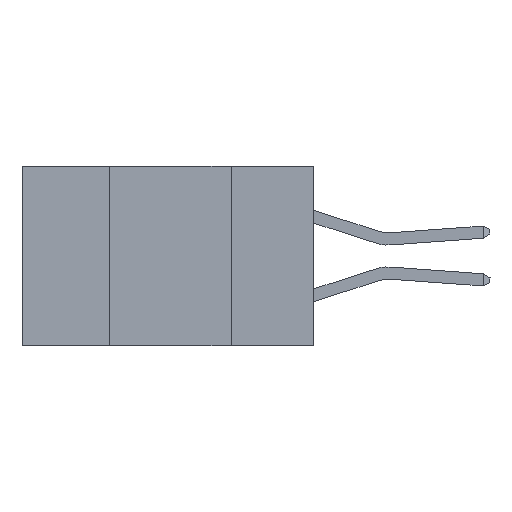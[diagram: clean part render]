
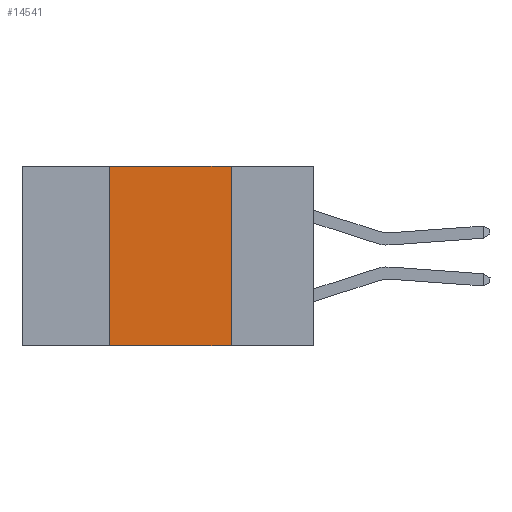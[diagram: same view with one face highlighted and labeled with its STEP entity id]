
A CAD part, left-side view. The second image highlights one B-rep face of the part: STEP entity #14541.
In plain terms, the highlighted planar face has unit normal (-1, 0, 0).
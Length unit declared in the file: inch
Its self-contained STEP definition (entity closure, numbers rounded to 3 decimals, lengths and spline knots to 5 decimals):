
#114 = CARTESIAN_POINT ( 'NONE',  ( 0., 0.42, 0. ) ) ;
#957 = CARTESIAN_POINT ( 'NONE',  ( 0., 0.6, 0. ) ) ;
#1025 = LINE ( 'NONE', #11012, #9658 ) ;
#1291 = VECTOR ( 'NONE', #13780, 39.37008 ) ;
#1461 = DIRECTION ( 'NONE',  ( 0., 0., -1. ) ) ;
#3761 = LINE ( 'NONE', #13973, #9531 ) ;
#5796 = EDGE_CURVE ( 'NONE', #7577, #7219, #10593, .T. ) ;
#5825 = DIRECTION ( 'NONE',  ( 1., 0., 0. ) ) ;
#6589 = EDGE_CURVE ( 'NONE', #7577, #11306, #13295, .T. ) ;
#7219 = VERTEX_POINT ( 'NONE', #9376 ) ;
#7380 = EDGE_CURVE ( 'NONE', #11321, #7219, #3761, .T. ) ;
#7577 = VERTEX_POINT ( 'NONE', #10891 ) ;
#7833 = CARTESIAN_POINT ( 'NONE',  ( 0., 0.42, 0. ) ) ;
#8542 = DIRECTION ( 'NONE',  ( 0., 0., 1. ) ) ;
#8641 = AXIS2_PLACEMENT_3D ( 'NONE', #957, #5825, #13574 ) ;
#8946 = CARTESIAN_POINT ( 'NONE',  ( 0., 0.17, 0. ) ) ;
#9052 = EDGE_CURVE ( 'NONE', #11306, #11321, #1025, .T. ) ;
#9376 = CARTESIAN_POINT ( 'NONE',  ( 0., 0.17, -0.37 ) ) ;
#9531 = VECTOR ( 'NONE', #1461, 39.37008 ) ;
#9658 = VECTOR ( 'NONE', #14293, 39.37008 ) ;
#10530 = CARTESIAN_POINT ( 'NONE',  ( 0., 0.6, -0.37 ) ) ;
#10593 = LINE ( 'NONE', #10530, #1291 ) ;
#10736 = VECTOR ( 'NONE', #8542, 39.37008 ) ;
#10891 = CARTESIAN_POINT ( 'NONE',  ( 0., 0.42, -0.37 ) ) ;
#10918 = FACE_OUTER_BOUND ( 'NONE', #11100, .T. ) ;
#11012 = CARTESIAN_POINT ( 'NONE',  ( 0., 0.6, 0. ) ) ;
#11100 = EDGE_LOOP ( 'NONE', ( #11796, #13339, #12402, #13402 ) ) ;
#11306 = VERTEX_POINT ( 'NONE', #7833 ) ;
#11321 = VERTEX_POINT ( 'NONE', #8946 ) ;
#11355 = PLANE ( 'NONE',  #8641 ) ;
#11796 = ORIENTED_EDGE ( 'NONE', *, *, #7380, .F. ) ;
#12402 = ORIENTED_EDGE ( 'NONE', *, *, #6589, .F. ) ;
#13295 = LINE ( 'NONE', #114, #10736 ) ;
#13339 = ORIENTED_EDGE ( 'NONE', *, *, #9052, .F. ) ;
#13402 = ORIENTED_EDGE ( 'NONE', *, *, #5796, .T. ) ;
#13574 = DIRECTION ( 'NONE',  ( 0., 0., -1. ) ) ;
#13780 = DIRECTION ( 'NONE',  ( 0., -1., 0. ) ) ;
#13973 = CARTESIAN_POINT ( 'NONE',  ( 0., 0.17, 0. ) ) ;
#14293 = DIRECTION ( 'NONE',  ( 0., -1., 0. ) ) ;
#14541 = ADVANCED_FACE ( 'NONE', ( #10918 ), #11355, .F. ) ;
